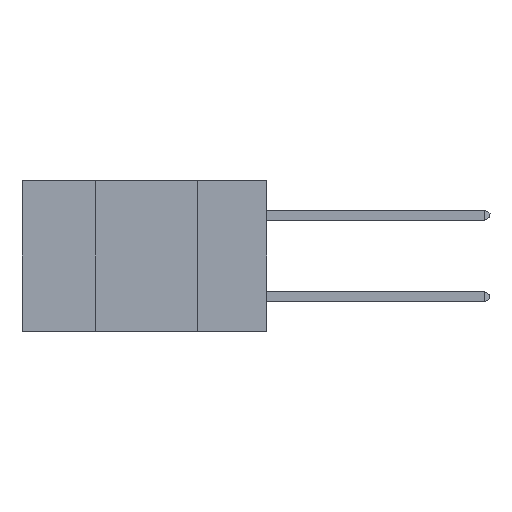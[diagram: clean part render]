
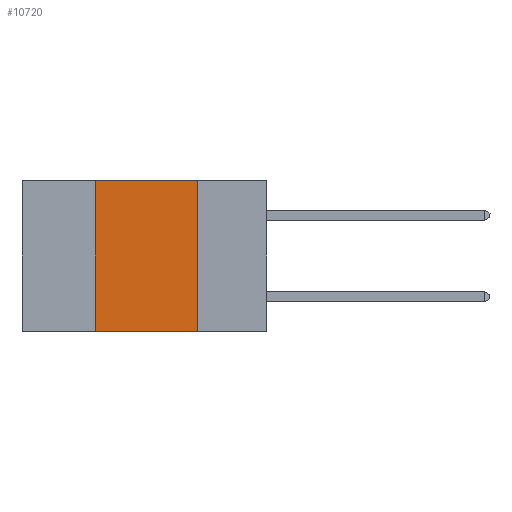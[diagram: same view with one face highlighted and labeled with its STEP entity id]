
A CAD part, left-side view. The second image highlights one B-rep face of the part: STEP entity #10720.
In plain terms, the highlighted planar face has unit normal (-1, 0, 0).
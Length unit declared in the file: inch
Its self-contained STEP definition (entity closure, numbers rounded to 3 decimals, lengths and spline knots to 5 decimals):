
#838 = VERTEX_POINT ( 'NONE', #4229 ) ;
#960 = DIRECTION ( 'NONE',  ( 1., 0., 0. ) ) ;
#1529 = EDGE_CURVE ( 'NONE', #10275, #10370, #3572, .T. ) ;
#1832 = LINE ( 'NONE', #10287, #4171 ) ;
#1999 = CARTESIAN_POINT ( 'NONE',  ( 0., 0.6, 0. ) ) ;
#2057 = PLANE ( 'NONE',  #9083 ) ;
#2285 = CARTESIAN_POINT ( 'NONE',  ( 0., 0.42, 0. ) ) ;
#2829 = CARTESIAN_POINT ( 'NONE',  ( 0., 0.42, 0. ) ) ;
#3154 = EDGE_LOOP ( 'NONE', ( #8543, #8010, #3284, #9918 ) ) ;
#3209 = LINE ( 'NONE', #2285, #7458 ) ;
#3284 = ORIENTED_EDGE ( 'NONE', *, *, #6209, .F. ) ;
#3572 = LINE ( 'NONE', #3948, #11448 ) ;
#3818 = LINE ( 'NONE', #10233, #10754 ) ;
#3948 = CARTESIAN_POINT ( 'NONE',  ( 0., 0.6, 0. ) ) ;
#4171 = VECTOR ( 'NONE', #4560, 39.37008 ) ;
#4229 = CARTESIAN_POINT ( 'NONE',  ( 0., 0.17, -0.37 ) ) ;
#4560 = DIRECTION ( 'NONE',  ( 0., -1., 0. ) ) ;
#4894 = DIRECTION ( 'NONE',  ( 0., -1., 0. ) ) ;
#5068 = EDGE_CURVE ( 'NONE', #10370, #838, #3818, .T. ) ;
#6209 = EDGE_CURVE ( 'NONE', #7909, #10275, #3209, .T. ) ;
#7458 = VECTOR ( 'NONE', #11394, 39.37008 ) ;
#7550 = DIRECTION ( 'NONE',  ( 0., 0., -1. ) ) ;
#7909 = VERTEX_POINT ( 'NONE', #10694 ) ;
#8010 = ORIENTED_EDGE ( 'NONE', *, *, #1529, .F. ) ;
#8210 = EDGE_CURVE ( 'NONE', #7909, #838, #1832, .T. ) ;
#8428 = FACE_OUTER_BOUND ( 'NONE', #3154, .T. ) ;
#8543 = ORIENTED_EDGE ( 'NONE', *, *, #5068, .F. ) ;
#8554 = DIRECTION ( 'NONE',  ( 0., 0., -1. ) ) ;
#9083 = AXIS2_PLACEMENT_3D ( 'NONE', #1999, #960, #8554 ) ;
#9918 = ORIENTED_EDGE ( 'NONE', *, *, #8210, .T. ) ;
#10233 = CARTESIAN_POINT ( 'NONE',  ( 0., 0.17, 0. ) ) ;
#10275 = VERTEX_POINT ( 'NONE', #2829 ) ;
#10287 = CARTESIAN_POINT ( 'NONE',  ( 0., 0.6, -0.37 ) ) ;
#10370 = VERTEX_POINT ( 'NONE', #11068 ) ;
#10694 = CARTESIAN_POINT ( 'NONE',  ( 0., 0.42, -0.37 ) ) ;
#10720 = ADVANCED_FACE ( 'NONE', ( #8428 ), #2057, .F. ) ;
#10754 = VECTOR ( 'NONE', #7550, 39.37008 ) ;
#11068 = CARTESIAN_POINT ( 'NONE',  ( 0., 0.17, 0. ) ) ;
#11394 = DIRECTION ( 'NONE',  ( 0., 0., 1. ) ) ;
#11448 = VECTOR ( 'NONE', #4894, 39.37008 ) ;
